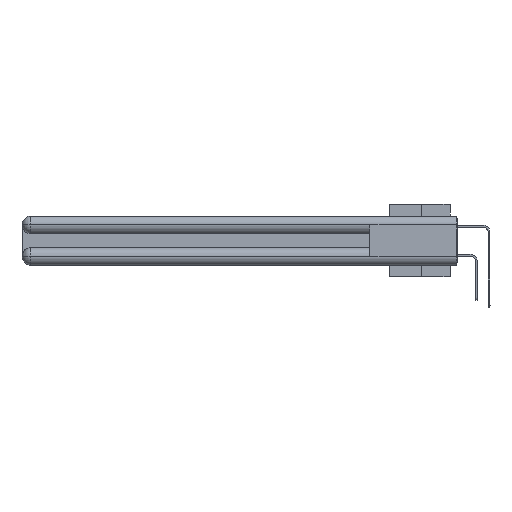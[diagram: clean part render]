
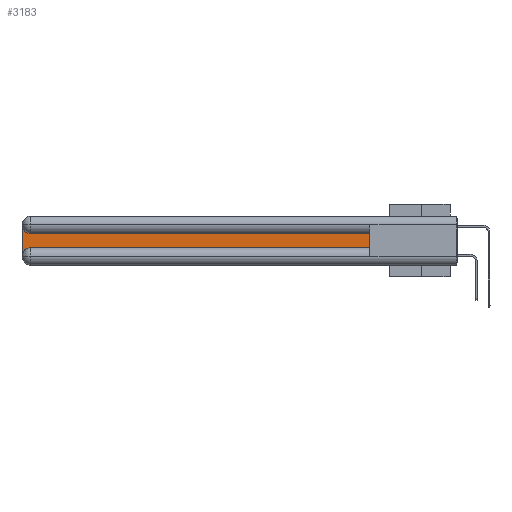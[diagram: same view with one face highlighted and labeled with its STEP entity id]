
A CAD part, left-side view. The second image highlights one B-rep face of the part: STEP entity #3183.
In plain terms, the highlighted planar face has unit normal (-1, 0, 0).
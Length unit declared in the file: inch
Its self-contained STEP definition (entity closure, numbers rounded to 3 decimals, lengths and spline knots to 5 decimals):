
#1101 = CARTESIAN_POINT ( 'NONE',  ( 0.075, 0.6, -0.2175 ) ) ;
#1116 = DIRECTION ( 'NONE',  ( 0., 0., -1. ) ) ;
#1521 = VECTOR ( 'NONE', #31958, 39.37008 ) ;
#1594 = LINE ( 'NONE', #26110, #7992 ) ;
#1623 = LINE ( 'NONE', #31601, #1521 ) ;
#1709 = DIRECTION ( 'NONE',  ( 1., 0., 0. ) ) ;
#2488 = ORIENTED_EDGE ( 'NONE', *, *, #10464, .T. ) ;
#3138 = PLANE ( 'NONE',  #11359 ) ;
#3183 = ADVANCED_FACE ( 'NONE', ( #19626 ), #3138, .F. ) ;
#3488 = CARTESIAN_POINT ( 'NONE',  ( 0.075, 2.94, -0.2775 ) ) ;
#4373 = VECTOR ( 'NONE', #31949, 39.37008 ) ;
#4673 = VERTEX_POINT ( 'NONE', #29789 ) ;
#4689 = DIRECTION ( 'NONE',  ( 0., 0., -1. ) ) ;
#6020 = EDGE_CURVE ( 'NONE', #18365, #4673, #33532, .T. ) ;
#6518 = EDGE_CURVE ( 'NONE', #4673, #27101, #18619, .T. ) ;
#7799 = EDGE_CURVE ( 'NONE', #19142, #18365, #1594, .T. ) ;
#7992 = VECTOR ( 'NONE', #26644, 39.37008 ) ;
#8926 = AXIS2_PLACEMENT_3D ( 'NONE', #3488, #9157, #1116 ) ;
#9157 = DIRECTION ( 'NONE',  ( 1., 0., 0. ) ) ;
#9564 = AXIS2_PLACEMENT_3D ( 'NONE', #15598, #1709, #29850 ) ;
#10464 = EDGE_CURVE ( 'NONE', #27101, #33105, #31129, .T. ) ;
#11359 = AXIS2_PLACEMENT_3D ( 'NONE', #27653, #17026, #33490 ) ;
#11621 = ORIENTED_EDGE ( 'NONE', *, *, #6020, .T. ) ;
#12585 = CARTESIAN_POINT ( 'NONE',  ( 0.075, 0.6, -0.2175 ) ) ;
#13358 = CARTESIAN_POINT ( 'NONE',  ( 0.075, 0.6, -0.1225 ) ) ;
#13432 = CARTESIAN_POINT ( 'NONE',  ( 0.075, 3., -0.2775 ) ) ;
#15598 = CARTESIAN_POINT ( 'NONE',  ( 0.075, 2.94, -0.0625 ) ) ;
#15736 = ORIENTED_EDGE ( 'NONE', *, *, #6518, .T. ) ;
#17026 = DIRECTION ( 'NONE',  ( 1., 0., 0. ) ) ;
#17340 = VECTOR ( 'NONE', #4689, 39.37008 ) ;
#18365 = VERTEX_POINT ( 'NONE', #25164 ) ;
#18619 = LINE ( 'NONE', #24470, #17340 ) ;
#19142 = VERTEX_POINT ( 'NONE', #13358 ) ;
#19238 = ORIENTED_EDGE ( 'NONE', *, *, #21298, .T. ) ;
#19626 = FACE_OUTER_BOUND ( 'NONE', #23534, .T. ) ;
#21298 = EDGE_CURVE ( 'NONE', #23869, #19142, #28685, .T. ) ;
#21345 = CARTESIAN_POINT ( 'NONE',  ( 0.075, 2.94, -0.2175 ) ) ;
#22558 = EDGE_CURVE ( 'NONE', #33105, #23869, #1623, .T. ) ;
#23534 = EDGE_LOOP ( 'NONE', ( #29446, #11621, #15736, #2488, #35929, #19238 ) ) ;
#23869 = VERTEX_POINT ( 'NONE', #1101 ) ;
#24470 = CARTESIAN_POINT ( 'NONE',  ( 0.075, 3., -0.2175 ) ) ;
#25164 = CARTESIAN_POINT ( 'NONE',  ( 0.075, 2.94, -0.1225 ) ) ;
#26110 = CARTESIAN_POINT ( 'NONE',  ( 0.075, 0.6, -0.1225 ) ) ;
#26644 = DIRECTION ( 'NONE',  ( 0., 1., 0. ) ) ;
#27101 = VERTEX_POINT ( 'NONE', #13432 ) ;
#27653 = CARTESIAN_POINT ( 'NONE',  ( 0.075, 3., -0.1225 ) ) ;
#28685 = LINE ( 'NONE', #12585, #4373 ) ;
#29446 = ORIENTED_EDGE ( 'NONE', *, *, #7799, .T. ) ;
#29789 = CARTESIAN_POINT ( 'NONE',  ( 0.075, 3., -0.0625 ) ) ;
#29850 = DIRECTION ( 'NONE',  ( 0., 0., -1. ) ) ;
#31129 = CIRCLE ( 'NONE', #8926, 0.06 ) ;
#31601 = CARTESIAN_POINT ( 'NONE',  ( 0.075, 0.6, -0.2175 ) ) ;
#31949 = DIRECTION ( 'NONE',  ( 0., 0., 1. ) ) ;
#31958 = DIRECTION ( 'NONE',  ( 0., -1., 0. ) ) ;
#33105 = VERTEX_POINT ( 'NONE', #21345 ) ;
#33490 = DIRECTION ( 'NONE',  ( 0., 0., -1. ) ) ;
#33532 = CIRCLE ( 'NONE', #9564, 0.06 ) ;
#35929 = ORIENTED_EDGE ( 'NONE', *, *, #22558, .T. ) ;
